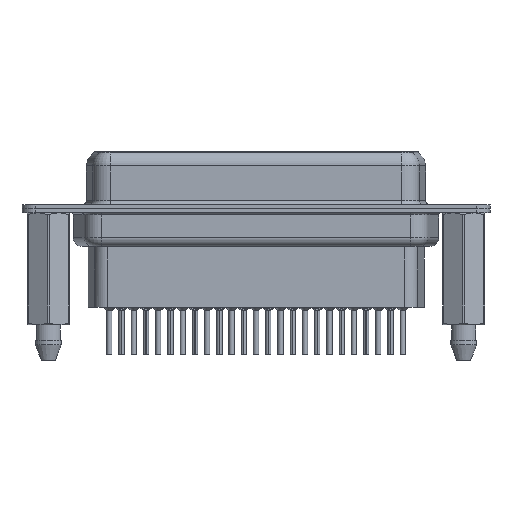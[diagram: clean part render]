
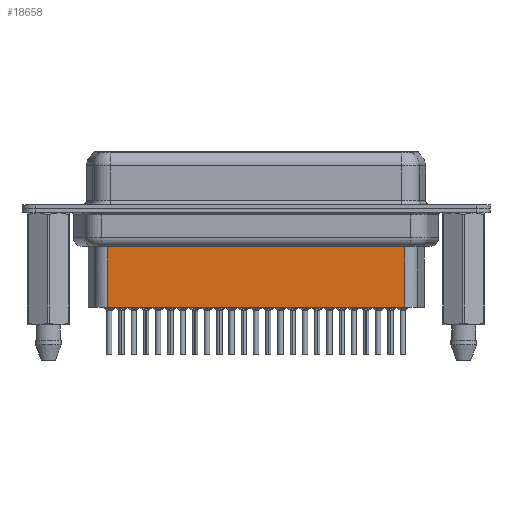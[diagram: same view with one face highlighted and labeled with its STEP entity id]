
A CAD part, front view. The second image highlights one B-rep face of the part: STEP entity #18658.
In plain terms, the highlighted planar face has unit normal (0, -1, 0).
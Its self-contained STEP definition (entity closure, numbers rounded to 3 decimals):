
#200 = LINE ( 'NONE', #6718, #24638 ) ;
#2036 = EDGE_CURVE ( 'NONE', #14733, #3990, #22713, .T. ) ;
#2487 = DIRECTION ( 'NONE',  ( 1., 0., 0. ) ) ;
#3990 = VERTEX_POINT ( 'NONE', #23770 ) ;
#4694 = FACE_OUTER_BOUND ( 'NONE', #25231, .T. ) ;
#5861 = VECTOR ( 'NONE', #15222, 1000. ) ;
#6563 = DIRECTION ( 'NONE',  ( 0., 0., -1. ) ) ;
#6718 = CARTESIAN_POINT ( 'NONE',  ( 6.706, -3.5, -3.1 ) ) ;
#6723 = DIRECTION ( 'NONE',  ( -1., 0., 0. ) ) ;
#8779 = CARTESIAN_POINT ( 'NONE',  ( 6.706, -3.5, -11.15 ) ) ;
#11011 = DIRECTION ( 'NONE',  ( 0., -1., 0. ) ) ;
#11110 = LINE ( 'NONE', #8779, #25990 ) ;
#12332 = ORIENTED_EDGE ( 'NONE', *, *, #2036, .T. ) ;
#13319 = VERTEX_POINT ( 'NONE', #25360 ) ;
#13507 = ORIENTED_EDGE ( 'NONE', *, *, #26910, .T. ) ;
#13655 = PLANE ( 'NONE',  #18079 ) ;
#14364 = VECTOR ( 'NONE', #20371, 1000. ) ;
#14451 = EDGE_CURVE ( 'NONE', #27032, #13319, #11110, .T. ) ;
#14663 = ORIENTED_EDGE ( 'NONE', *, *, #26331, .F. ) ;
#14733 = VERTEX_POINT ( 'NONE', #23887 ) ;
#15222 = DIRECTION ( 'NONE',  ( 0., 0., -1. ) ) ;
#15524 = CARTESIAN_POINT ( 'NONE',  ( 40.344, -3.5, -3.1 ) ) ;
#16709 = ORIENTED_EDGE ( 'NONE', *, *, #14451, .F. ) ;
#18079 = AXIS2_PLACEMENT_3D ( 'NONE', #22629, #11011, #2487 ) ;
#18658 = ADVANCED_FACE ( 'NONE', ( #4694 ), #13655, .T. ) ;
#20371 = DIRECTION ( 'NONE',  ( -1., 0., 0. ) ) ;
#22562 = LINE ( 'NONE', #15524, #5861 ) ;
#22629 = CARTESIAN_POINT ( 'NONE',  ( 6.706, -3.5, -3.1 ) ) ;
#22713 = LINE ( 'NONE', #26993, #14364 ) ;
#22864 = CARTESIAN_POINT ( 'NONE',  ( 40.344, -3.5, -11.15 ) ) ;
#23770 = CARTESIAN_POINT ( 'NONE',  ( 6.706, -3.5, -4.097 ) ) ;
#23887 = CARTESIAN_POINT ( 'NONE',  ( 40.344, -3.5, -4.097 ) ) ;
#24638 = VECTOR ( 'NONE', #6563, 1000. ) ;
#25231 = EDGE_LOOP ( 'NONE', ( #14663, #12332, #13507, #16709 ) ) ;
#25360 = CARTESIAN_POINT ( 'NONE',  ( 6.706, -3.5, -11.15 ) ) ;
#25990 = VECTOR ( 'NONE', #6723, 1000. ) ;
#26331 = EDGE_CURVE ( 'NONE', #14733, #27032, #22562, .T. ) ;
#26910 = EDGE_CURVE ( 'NONE', #3990, #13319, #200, .T. ) ;
#26993 = CARTESIAN_POINT ( 'NONE',  ( 6.459, -3.5, -4.097 ) ) ;
#27032 = VERTEX_POINT ( 'NONE', #22864 ) ;
